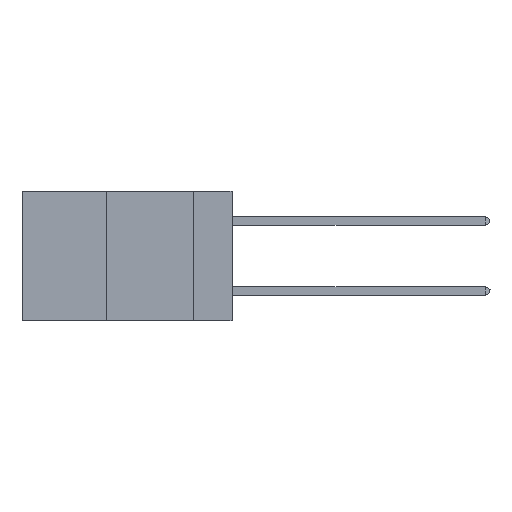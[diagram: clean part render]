
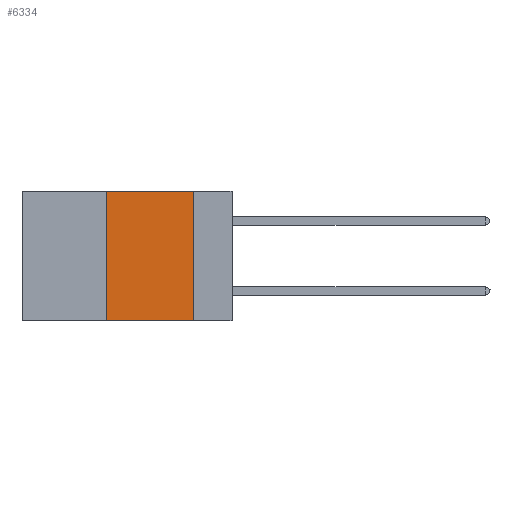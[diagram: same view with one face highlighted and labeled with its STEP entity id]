
A CAD part, left-side view. The second image highlights one B-rep face of the part: STEP entity #6334.
In plain terms, the highlighted planar face has unit normal (-1, 0, 0).
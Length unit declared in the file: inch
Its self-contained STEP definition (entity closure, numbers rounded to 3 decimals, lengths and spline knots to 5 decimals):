
#196 = VECTOR ( 'NONE', #9578, 39.37008 ) ;
#518 = VECTOR ( 'NONE', #765, 39.37008 ) ;
#765 = DIRECTION ( 'NONE',  ( 0., -1., 0. ) ) ;
#935 = VERTEX_POINT ( 'NONE', #5023 ) ;
#1556 = AXIS2_PLACEMENT_3D ( 'NONE', #10020, #10096, #11935 ) ;
#2413 = CARTESIAN_POINT ( 'NONE',  ( 0., 0.6, -0.37 ) ) ;
#2449 = CARTESIAN_POINT ( 'NONE',  ( 0., 0.11, -0.37 ) ) ;
#2506 = CARTESIAN_POINT ( 'NONE',  ( 0., 0.6, 0. ) ) ;
#3641 = EDGE_CURVE ( 'NONE', #935, #9814, #8873, .T. ) ;
#4037 = VERTEX_POINT ( 'NONE', #10169 ) ;
#4884 = DIRECTION ( 'NONE',  ( 0., 0., 1. ) ) ;
#4990 = VECTOR ( 'NONE', #8669, 39.37008 ) ;
#5023 = CARTESIAN_POINT ( 'NONE',  ( 0., 0.36, -0.37 ) ) ;
#5814 = ORIENTED_EDGE ( 'NONE', *, *, #11261, .F. ) ;
#5965 = LINE ( 'NONE', #2506, #518 ) ;
#6334 = ADVANCED_FACE ( 'NONE', ( #8975 ), #9020, .F. ) ;
#7553 = LINE ( 'NONE', #10625, #4990 ) ;
#7929 = CARTESIAN_POINT ( 'NONE',  ( 0., 0.36, 0. ) ) ;
#8669 = DIRECTION ( 'NONE',  ( 0., 0., -1. ) ) ;
#8809 = ORIENTED_EDGE ( 'NONE', *, *, #9457, .F. ) ;
#8873 = LINE ( 'NONE', #2413, #196 ) ;
#8975 = FACE_OUTER_BOUND ( 'NONE', #11703, .T. ) ;
#9020 = PLANE ( 'NONE',  #1556 ) ;
#9456 = VERTEX_POINT ( 'NONE', #7929 ) ;
#9457 = EDGE_CURVE ( 'NONE', #935, #9456, #9855, .T. ) ;
#9520 = VECTOR ( 'NONE', #4884, 39.37008 ) ;
#9578 = DIRECTION ( 'NONE',  ( 0., -1., 0. ) ) ;
#9814 = VERTEX_POINT ( 'NONE', #2449 ) ;
#9855 = LINE ( 'NONE', #13108, #9520 ) ;
#10020 = CARTESIAN_POINT ( 'NONE',  ( 0., 0.6, 0. ) ) ;
#10096 = DIRECTION ( 'NONE',  ( 1., 0., 0. ) ) ;
#10169 = CARTESIAN_POINT ( 'NONE',  ( 0., 0.11, 0. ) ) ;
#10625 = CARTESIAN_POINT ( 'NONE',  ( 0., 0.11, 0. ) ) ;
#10714 = ORIENTED_EDGE ( 'NONE', *, *, #11901, .F. ) ;
#11261 = EDGE_CURVE ( 'NONE', #4037, #9814, #7553, .T. ) ;
#11703 = EDGE_LOOP ( 'NONE', ( #5814, #10714, #8809, #12872 ) ) ;
#11901 = EDGE_CURVE ( 'NONE', #9456, #4037, #5965, .T. ) ;
#11935 = DIRECTION ( 'NONE',  ( 0., 0., -1. ) ) ;
#12872 = ORIENTED_EDGE ( 'NONE', *, *, #3641, .T. ) ;
#13108 = CARTESIAN_POINT ( 'NONE',  ( 0., 0.36, 0. ) ) ;
